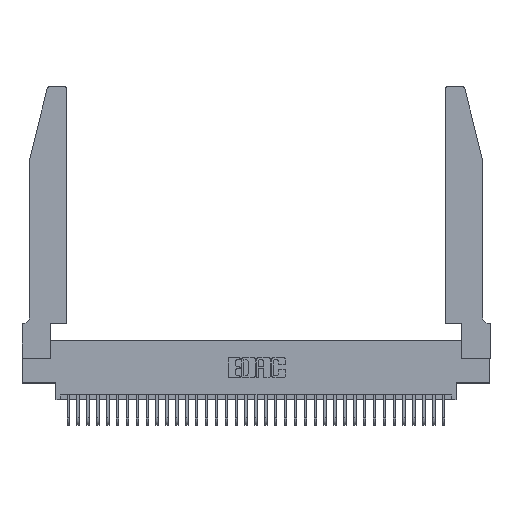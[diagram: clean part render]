
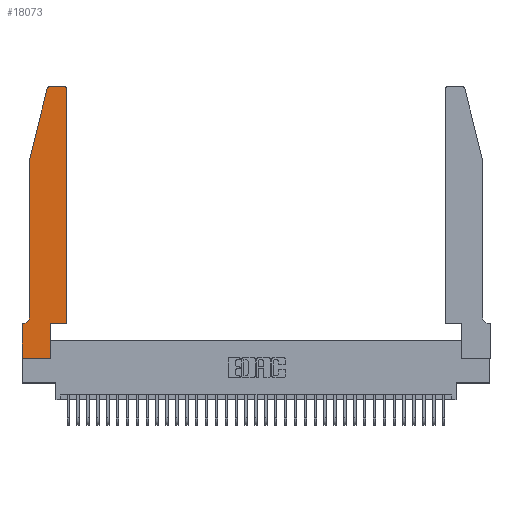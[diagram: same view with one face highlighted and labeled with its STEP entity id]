
A CAD part, top view. The second image highlights one B-rep face of the part: STEP entity #18073.
In plain terms, the highlighted planar face has unit normal (0, 0, 1).
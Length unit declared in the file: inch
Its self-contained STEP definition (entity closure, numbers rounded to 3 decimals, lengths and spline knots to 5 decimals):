
#117 = LINE ( 'NONE', #33167, #36874 ) ;
#287 = EDGE_LOOP ( 'NONE', ( #13743, #25960, #31451, #10011, #18067, #34586, #9663, #6502, #37421, #11176, #5827, #31965 ) ) ;
#289 = VECTOR ( 'NONE', #6158, 39.37008 ) ;
#601 = LINE ( 'NONE', #13513, #17050 ) ;
#710 = VECTOR ( 'NONE', #20901, 39.37008 ) ;
#786 = CARTESIAN_POINT ( 'NONE',  ( 0.4205, 2.75, 0.37 ) ) ;
#935 = CARTESIAN_POINT ( 'NONE',  ( 0.4505, 0.35, 0.37 ) ) ;
#1565 = VERTEX_POINT ( 'NONE', #15775 ) ;
#1905 = VECTOR ( 'NONE', #34288, 39.37008 ) ;
#2173 = AXIS2_PLACEMENT_3D ( 'NONE', #2796, #17597, #18640 ) ;
#2615 = CIRCLE ( 'NONE', #30406, 0.03 ) ;
#2684 = EDGE_CURVE ( 'NONE', #27854, #11032, #35137, .T. ) ;
#2796 = CARTESIAN_POINT ( 'NONE',  ( 0.0055, 0.42, 0.37 ) ) ;
#3073 = EDGE_CURVE ( 'NONE', #30707, #21185, #23946, .T. ) ;
#3364 = EDGE_CURVE ( 'NONE', #17389, #4185, #6210, .T. ) ;
#3717 = EDGE_CURVE ( 'NONE', #21185, #6455, #25771, .T. ) ;
#4185 = VERTEX_POINT ( 'NONE', #22468 ) ;
#4304 = CARTESIAN_POINT ( 'NONE',  ( 0., 0.35, 0.37 ) ) ;
#4604 = EDGE_CURVE ( 'NONE', #11032, #30636, #601, .T. ) ;
#5057 = CARTESIAN_POINT ( 'NONE',  ( 0.4505, 0.35, 0.37 ) ) ;
#5827 = ORIENTED_EDGE ( 'NONE', *, *, #20884, .T. ) ;
#5854 = DIRECTION ( 'NONE',  ( 0., 1., 0. ) ) ;
#6158 = DIRECTION ( 'NONE',  ( 1., 0., 0. ) ) ;
#6210 = LINE ( 'NONE', #36109, #710 ) ;
#6303 = CARTESIAN_POINT ( 'NONE',  ( 0.25487, 2.72718, 0.37 ) ) ;
#6393 = EDGE_CURVE ( 'NONE', #26871, #31515, #117, .T. ) ;
#6435 = CARTESIAN_POINT ( 'NONE',  ( 0., 0., 0.37 ) ) ;
#6455 = VERTEX_POINT ( 'NONE', #5057 ) ;
#6502 = ORIENTED_EDGE ( 'NONE', *, *, #29155, .T. ) ;
#7556 = DIRECTION ( 'NONE',  ( 0., 0., 1. ) ) ;
#9663 = ORIENTED_EDGE ( 'NONE', *, *, #27871, .T. ) ;
#9813 = DIRECTION ( 'NONE',  ( 0., 0., 1. ) ) ;
#10011 = ORIENTED_EDGE ( 'NONE', *, *, #17657, .T. ) ;
#10599 = DIRECTION ( 'NONE',  ( 0., -1., 0. ) ) ;
#10806 = CARTESIAN_POINT ( 'NONE',  ( 0.0755, 2., 0.37 ) ) ;
#11014 = LINE ( 'NONE', #14269, #1905 ) ;
#11032 = VERTEX_POINT ( 'NONE', #15586 ) ;
#11176 = ORIENTED_EDGE ( 'NONE', *, *, #3717, .T. ) ;
#11637 = LINE ( 'NONE', #25348, #12979 ) ;
#12665 = CARTESIAN_POINT ( 'NONE',  ( 0.2865, 0.35, 0.37 ) ) ;
#12979 = VECTOR ( 'NONE', #25208, 39.37008 ) ;
#13376 = DIRECTION ( 'NONE',  ( -1., 0., 0. ) ) ;
#13513 = CARTESIAN_POINT ( 'NONE',  ( 0.0755, 0.35, 0.37 ) ) ;
#13743 = ORIENTED_EDGE ( 'NONE', *, *, #3364, .T. ) ;
#14269 = CARTESIAN_POINT ( 'NONE',  ( 0.4505, 0.35, 0.37 ) ) ;
#15048 = LINE ( 'NONE', #6435, #27764 ) ;
#15461 = PLANE ( 'NONE',  #35431 ) ;
#15524 = CARTESIAN_POINT ( 'NONE',  ( 0.4205, 2.72, 0.37 ) ) ;
#15586 = CARTESIAN_POINT ( 'NONE',  ( 0.0055, 0.35, 0.37 ) ) ;
#15775 = CARTESIAN_POINT ( 'NONE',  ( 0.4505, 2.72, 0.37 ) ) ;
#15861 = DIRECTION ( 'NONE',  ( 1., 0., 0. ) ) ;
#16576 = CARTESIAN_POINT ( 'NONE',  ( 0., 0., 0.37 ) ) ;
#17050 = VECTOR ( 'NONE', #13376, 39.37008 ) ;
#17075 = FACE_OUTER_BOUND ( 'NONE', #287, .T. ) ;
#17389 = VERTEX_POINT ( 'NONE', #786 ) ;
#17597 = DIRECTION ( 'NONE',  ( 0., 0., -1. ) ) ;
#17657 = EDGE_CURVE ( 'NONE', #31515, #27854, #11637, .T. ) ;
#18067 = ORIENTED_EDGE ( 'NONE', *, *, #2684, .T. ) ;
#18073 = ADVANCED_FACE ( 'NONE', ( #17075 ), #15461, .T. ) ;
#18640 = DIRECTION ( 'NONE',  ( -1., 0., 0. ) ) ;
#18718 = DIRECTION ( 'NONE',  ( 1., 0., 0. ) ) ;
#19022 = DIRECTION ( 'NONE',  ( -0.239, -0.971, 0. ) ) ;
#19201 = DIRECTION ( 'NONE',  ( 0., 0., 1. ) ) ;
#19422 = CARTESIAN_POINT ( 'NONE',  ( 0., 0., 0.37 ) ) ;
#19939 = EDGE_CURVE ( 'NONE', #1565, #17389, #31499, .T. ) ;
#20884 = EDGE_CURVE ( 'NONE', #6455, #1565, #11014, .T. ) ;
#20901 = DIRECTION ( 'NONE',  ( -1., 0., 0. ) ) ;
#21170 = CARTESIAN_POINT ( 'NONE',  ( 0.2865, 0.35, 0.37 ) ) ;
#21185 = VERTEX_POINT ( 'NONE', #21170 ) ;
#22468 = CARTESIAN_POINT ( 'NONE',  ( 0.284, 2.75, 0.37 ) ) ;
#22659 = CARTESIAN_POINT ( 'NONE',  ( 0., 0.35, 0.37 ) ) ;
#23317 = DIRECTION ( 'NONE',  ( 1., 0., 0. ) ) ;
#23946 = LINE ( 'NONE', #12665, #24898 ) ;
#24583 = AXIS2_PLACEMENT_3D ( 'NONE', #15524, #9813, #18718 ) ;
#24898 = VECTOR ( 'NONE', #5854, 39.37008 ) ;
#25208 = DIRECTION ( 'NONE',  ( 0., -1., 0. ) ) ;
#25348 = CARTESIAN_POINT ( 'NONE',  ( 0.0755, 2., 0.37 ) ) ;
#25476 = CARTESIAN_POINT ( 'NONE',  ( 0.2865, 0., 0.37 ) ) ;
#25541 = VERTEX_POINT ( 'NONE', #19422 ) ;
#25771 = LINE ( 'NONE', #935, #289 ) ;
#25960 = ORIENTED_EDGE ( 'NONE', *, *, #36434, .T. ) ;
#26871 = VERTEX_POINT ( 'NONE', #6303 ) ;
#27764 = VECTOR ( 'NONE', #15861, 39.37008 ) ;
#27854 = VERTEX_POINT ( 'NONE', #33917 ) ;
#27871 = EDGE_CURVE ( 'NONE', #30636, #25541, #35539, .T. ) ;
#29155 = EDGE_CURVE ( 'NONE', #25541, #30707, #15048, .T. ) ;
#29235 = VECTOR ( 'NONE', #10599, 39.37008 ) ;
#30406 = AXIS2_PLACEMENT_3D ( 'NONE', #36625, #7556, #36483 ) ;
#30636 = VERTEX_POINT ( 'NONE', #22659 ) ;
#30707 = VERTEX_POINT ( 'NONE', #25476 ) ;
#31451 = ORIENTED_EDGE ( 'NONE', *, *, #6393, .T. ) ;
#31499 = CIRCLE ( 'NONE', #24583, 0.03 ) ;
#31515 = VERTEX_POINT ( 'NONE', #10806 ) ;
#31965 = ORIENTED_EDGE ( 'NONE', *, *, #19939, .T. ) ;
#33167 = CARTESIAN_POINT ( 'NONE',  ( 0.0755, 2., 0.37 ) ) ;
#33917 = CARTESIAN_POINT ( 'NONE',  ( 0.0755, 0.42, 0.37 ) ) ;
#34288 = DIRECTION ( 'NONE',  ( 0., 1., 0. ) ) ;
#34586 = ORIENTED_EDGE ( 'NONE', *, *, #4604, .T. ) ;
#35137 = CIRCLE ( 'NONE', #2173, 0.07 ) ;
#35431 = AXIS2_PLACEMENT_3D ( 'NONE', #4304, #19201, #23317 ) ;
#35539 = LINE ( 'NONE', #16576, #29235 ) ;
#36109 = CARTESIAN_POINT ( 'NONE',  ( 0.2605, 2.75, 0.37 ) ) ;
#36434 = EDGE_CURVE ( 'NONE', #4185, #26871, #2615, .T. ) ;
#36483 = DIRECTION ( 'NONE',  ( 1., 0., 0. ) ) ;
#36625 = CARTESIAN_POINT ( 'NONE',  ( 0.284, 2.72, 0.37 ) ) ;
#36874 = VECTOR ( 'NONE', #19022, 39.37008 ) ;
#37421 = ORIENTED_EDGE ( 'NONE', *, *, #3073, .T. ) ;
